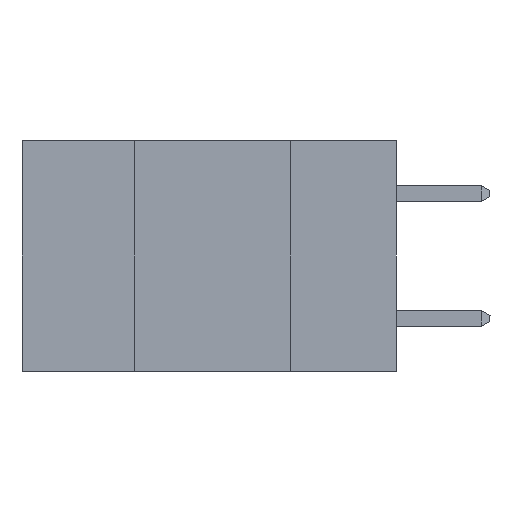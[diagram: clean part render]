
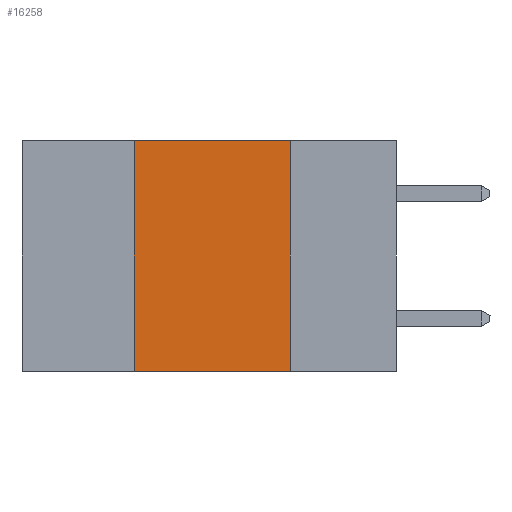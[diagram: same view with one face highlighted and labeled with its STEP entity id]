
A CAD part, left-side view. The second image highlights one B-rep face of the part: STEP entity #16258.
In plain terms, the highlighted planar face has unit normal (-1, 0, 0).
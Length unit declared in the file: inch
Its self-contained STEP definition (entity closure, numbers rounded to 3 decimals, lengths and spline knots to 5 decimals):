
#523 = VECTOR ( 'NONE', #26828, 39.37008 ) ;
#2413 = EDGE_CURVE ( 'NONE', #11889, #17610, #7189, .T. ) ;
#2649 = LINE ( 'NONE', #9224, #6949 ) ;
#2882 = CARTESIAN_POINT ( 'NONE',  ( 0., 0.42, 0. ) ) ;
#4514 = ORIENTED_EDGE ( 'NONE', *, *, #2413, .F. ) ;
#4715 = AXIS2_PLACEMENT_3D ( 'NONE', #21431, #13970, #31010 ) ;
#5807 = LINE ( 'NONE', #25759, #20917 ) ;
#6614 = CARTESIAN_POINT ( 'NONE',  ( 0., 0.42, 0. ) ) ;
#6949 = VECTOR ( 'NONE', #26515, 39.37008 ) ;
#7189 = LINE ( 'NONE', #6614, #523 ) ;
#8888 = PLANE ( 'NONE',  #4715 ) ;
#9224 = CARTESIAN_POINT ( 'NONE',  ( 0., 0.17, 0. ) ) ;
#9757 = VERTEX_POINT ( 'NONE', #21351 ) ;
#10247 = FACE_OUTER_BOUND ( 'NONE', #17683, .T. ) ;
#11889 = VERTEX_POINT ( 'NONE', #29947 ) ;
#12987 = EDGE_CURVE ( 'NONE', #9757, #22917, #2649, .T. ) ;
#13199 = ORIENTED_EDGE ( 'NONE', *, *, #18853, .F. ) ;
#13970 = DIRECTION ( 'NONE',  ( 1., 0., 0. ) ) ;
#15674 = LINE ( 'NONE', #23517, #18373 ) ;
#16202 = EDGE_CURVE ( 'NONE', #11889, #22917, #15674, .T. ) ;
#16258 = ADVANCED_FACE ( 'NONE', ( #10247 ), #8888, .F. ) ;
#17610 = VERTEX_POINT ( 'NONE', #2882 ) ;
#17683 = EDGE_LOOP ( 'NONE', ( #30426, #13199, #4514, #20469 ) ) ;
#18373 = VECTOR ( 'NONE', #25958, 39.37008 ) ;
#18853 = EDGE_CURVE ( 'NONE', #17610, #9757, #5807, .T. ) ;
#20469 = ORIENTED_EDGE ( 'NONE', *, *, #16202, .T. ) ;
#20917 = VECTOR ( 'NONE', #21023, 39.37008 ) ;
#21023 = DIRECTION ( 'NONE',  ( 0., -1., 0. ) ) ;
#21351 = CARTESIAN_POINT ( 'NONE',  ( 0., 0.17, 0. ) ) ;
#21431 = CARTESIAN_POINT ( 'NONE',  ( 0., 0.6, 0. ) ) ;
#22917 = VERTEX_POINT ( 'NONE', #25443 ) ;
#23517 = CARTESIAN_POINT ( 'NONE',  ( 0., 0.6, -0.37 ) ) ;
#25443 = CARTESIAN_POINT ( 'NONE',  ( 0., 0.17, -0.37 ) ) ;
#25759 = CARTESIAN_POINT ( 'NONE',  ( 0., 0.6, 0. ) ) ;
#25958 = DIRECTION ( 'NONE',  ( 0., -1., 0. ) ) ;
#26515 = DIRECTION ( 'NONE',  ( 0., 0., -1. ) ) ;
#26828 = DIRECTION ( 'NONE',  ( 0., 0., 1. ) ) ;
#29947 = CARTESIAN_POINT ( 'NONE',  ( 0., 0.42, -0.37 ) ) ;
#30426 = ORIENTED_EDGE ( 'NONE', *, *, #12987, .F. ) ;
#31010 = DIRECTION ( 'NONE',  ( 0., 0., -1. ) ) ;
